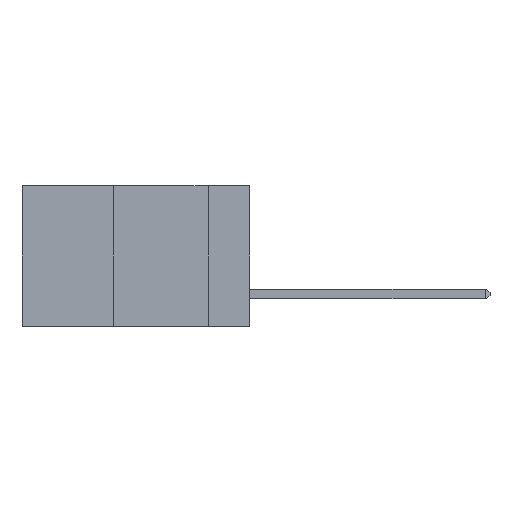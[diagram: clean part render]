
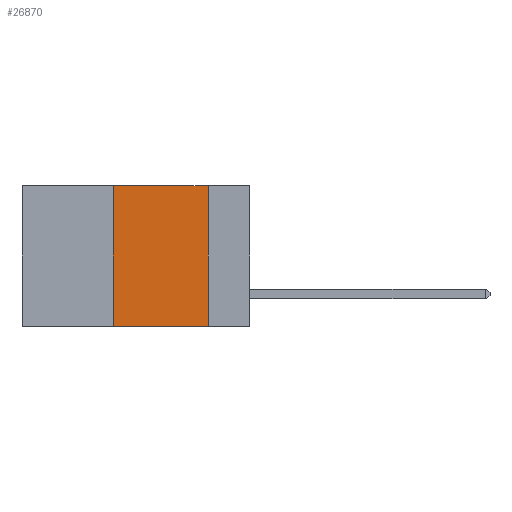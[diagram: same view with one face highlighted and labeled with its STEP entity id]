
A CAD part, left-side view. The second image highlights one B-rep face of the part: STEP entity #26870.
In plain terms, the highlighted planar face has unit normal (-1, 0, 0).
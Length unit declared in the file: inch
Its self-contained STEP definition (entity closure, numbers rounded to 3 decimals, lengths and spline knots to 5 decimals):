
#142 = EDGE_CURVE ( 'NONE', #9332, #13135, #184, .T. ) ;
#184 = LINE ( 'NONE', #14435, #11789 ) ;
#998 = EDGE_LOOP ( 'NONE', ( #16592, #16027, #12958, #22058 ) ) ;
#1498 = VECTOR ( 'NONE', #4475, 39.37008 ) ;
#2021 = DIRECTION ( 'NONE',  ( 0., -1., 0. ) ) ;
#4475 = DIRECTION ( 'NONE',  ( 0., 0., -1. ) ) ;
#5616 = VERTEX_POINT ( 'NONE', #11800 ) ;
#5919 = CARTESIAN_POINT ( 'NONE',  ( 0., 0.36, 0. ) ) ;
#7290 = LINE ( 'NONE', #19573, #1498 ) ;
#7340 = DIRECTION ( 'NONE',  ( 1., 0., 0. ) ) ;
#9332 = VERTEX_POINT ( 'NONE', #18669 ) ;
#10226 = DIRECTION ( 'NONE',  ( 0., 0., 1. ) ) ;
#11024 = EDGE_CURVE ( 'NONE', #19831, #5616, #11634, .T. ) ;
#11634 = LINE ( 'NONE', #12927, #19021 ) ;
#11789 = VECTOR ( 'NONE', #20802, 39.37008 ) ;
#11800 = CARTESIAN_POINT ( 'NONE',  ( 0., 0.11, 0. ) ) ;
#12202 = CARTESIAN_POINT ( 'NONE',  ( 0., 0.11, -0.37 ) ) ;
#12495 = AXIS2_PLACEMENT_3D ( 'NONE', #20327, #7340, #22506 ) ;
#12927 = CARTESIAN_POINT ( 'NONE',  ( 0., 0.6, 0. ) ) ;
#12958 = ORIENTED_EDGE ( 'NONE', *, *, #16200, .F. ) ;
#13135 = VERTEX_POINT ( 'NONE', #12202 ) ;
#14435 = CARTESIAN_POINT ( 'NONE',  ( 0., 0.6, -0.37 ) ) ;
#15058 = LINE ( 'NONE', #5919, #26409 ) ;
#16027 = ORIENTED_EDGE ( 'NONE', *, *, #11024, .F. ) ;
#16200 = EDGE_CURVE ( 'NONE', #9332, #19831, #15058, .T. ) ;
#16592 = ORIENTED_EDGE ( 'NONE', *, *, #20528, .F. ) ;
#16673 = FACE_OUTER_BOUND ( 'NONE', #998, .T. ) ;
#18170 = PLANE ( 'NONE',  #12495 ) ;
#18669 = CARTESIAN_POINT ( 'NONE',  ( 0., 0.36, -0.37 ) ) ;
#19021 = VECTOR ( 'NONE', #2021, 39.37008 ) ;
#19573 = CARTESIAN_POINT ( 'NONE',  ( 0., 0.11, 0. ) ) ;
#19831 = VERTEX_POINT ( 'NONE', #27435 ) ;
#20327 = CARTESIAN_POINT ( 'NONE',  ( 0., 0.6, 0. ) ) ;
#20528 = EDGE_CURVE ( 'NONE', #5616, #13135, #7290, .T. ) ;
#20802 = DIRECTION ( 'NONE',  ( 0., -1., 0. ) ) ;
#22058 = ORIENTED_EDGE ( 'NONE', *, *, #142, .T. ) ;
#22506 = DIRECTION ( 'NONE',  ( 0., 0., -1. ) ) ;
#26409 = VECTOR ( 'NONE', #10226, 39.37008 ) ;
#26870 = ADVANCED_FACE ( 'NONE', ( #16673 ), #18170, .F. ) ;
#27435 = CARTESIAN_POINT ( 'NONE',  ( 0., 0.36, 0. ) ) ;
